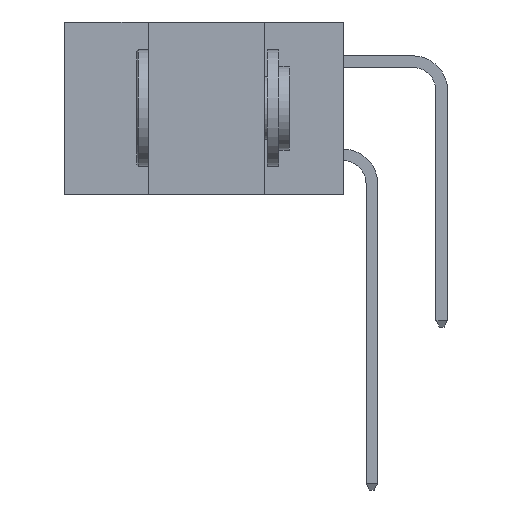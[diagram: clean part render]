
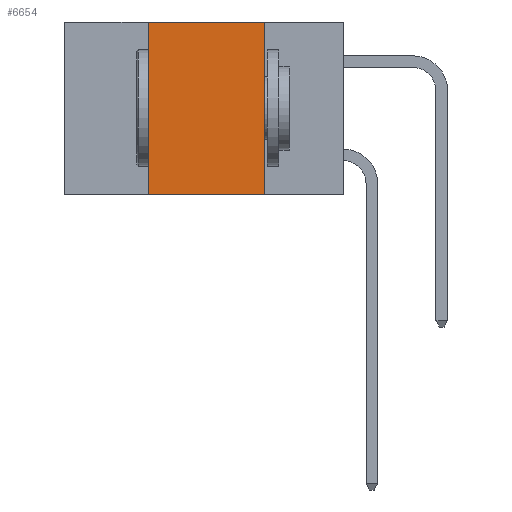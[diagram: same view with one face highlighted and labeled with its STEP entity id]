
A CAD part, left-side view. The second image highlights one B-rep face of the part: STEP entity #6654.
In plain terms, the highlighted planar face has unit normal (-1, 0, 0).
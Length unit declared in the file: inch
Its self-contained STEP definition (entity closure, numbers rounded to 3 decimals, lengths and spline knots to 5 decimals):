
#30 = DIRECTION ( 'NONE',  ( 0., 0., -1. ) ) ;
#78 = DIRECTION ( 'NONE',  ( 0., 0., -1. ) ) ;
#98 = DIRECTION ( 'NONE',  ( 1., 0., 0. ) ) ;
#119 = CARTESIAN_POINT ( 'NONE',  ( 0., 0.6, 0. ) ) ;
#271 = EDGE_LOOP ( 'NONE', ( #14424, #1793, #6080, #1649 ) ) ;
#317 = CARTESIAN_POINT ( 'NONE',  ( 0., 0.17, -0.37 ) ) ;
#319 = PLANE ( 'NONE',  #12376 ) ;
#1226 = LINE ( 'NONE', #317, #7999 ) ;
#1649 = ORIENTED_EDGE ( 'NONE', *, *, #15947, .T. ) ;
#1655 = VECTOR ( 'NONE', #17229, 39.37008 ) ;
#1793 = ORIENTED_EDGE ( 'NONE', *, *, #2169, .F. ) ;
#2169 = EDGE_CURVE ( 'NONE', #10352, #9445, #16256, .T. ) ;
#2186 = LINE ( 'NONE', #5900, #5558 ) ;
#2946 = CARTESIAN_POINT ( 'NONE',  ( 0., 0.42, -0.37 ) ) ;
#3409 = VERTEX_POINT ( 'NONE', #14683 ) ;
#5558 = VECTOR ( 'NONE', #14440, 39.37008 ) ;
#5900 = CARTESIAN_POINT ( 'NONE',  ( 0., 0.6, -0.37 ) ) ;
#6080 = ORIENTED_EDGE ( 'NONE', *, *, #17703, .F. ) ;
#6342 = CARTESIAN_POINT ( 'NONE',  ( 0., 0.17, 0. ) ) ;
#6654 = ADVANCED_FACE ( 'NONE', ( #12407 ), #319, .F. ) ;
#6978 = DIRECTION ( 'NONE',  ( 0., -1., 0. ) ) ;
#7999 = VECTOR ( 'NONE', #30, 39.37008 ) ;
#8189 = CARTESIAN_POINT ( 'NONE',  ( 0., 0.42, 0. ) ) ;
#8804 = CARTESIAN_POINT ( 'NONE',  ( 0., 0.6, 0. ) ) ;
#8834 = CARTESIAN_POINT ( 'NONE',  ( 0., 0.42, -0.37 ) ) ;
#9445 = VERTEX_POINT ( 'NONE', #6342 ) ;
#10352 = VERTEX_POINT ( 'NONE', #8189 ) ;
#12376 = AXIS2_PLACEMENT_3D ( 'NONE', #119, #98, #78 ) ;
#12407 = FACE_OUTER_BOUND ( 'NONE', #271, .T. ) ;
#12578 = VECTOR ( 'NONE', #6978, 39.37008 ) ;
#13709 = EDGE_CURVE ( 'NONE', #9445, #3409, #1226, .T. ) ;
#14025 = VERTEX_POINT ( 'NONE', #2946 ) ;
#14424 = ORIENTED_EDGE ( 'NONE', *, *, #13709, .F. ) ;
#14440 = DIRECTION ( 'NONE',  ( 0., -1., 0. ) ) ;
#14683 = CARTESIAN_POINT ( 'NONE',  ( 0., 0.17, -0.37 ) ) ;
#15947 = EDGE_CURVE ( 'NONE', #14025, #3409, #2186, .T. ) ;
#16256 = LINE ( 'NONE', #8804, #12578 ) ;
#16821 = LINE ( 'NONE', #8834, #1655 ) ;
#17229 = DIRECTION ( 'NONE',  ( 0., 0., 1. ) ) ;
#17703 = EDGE_CURVE ( 'NONE', #14025, #10352, #16821, .T. ) ;
